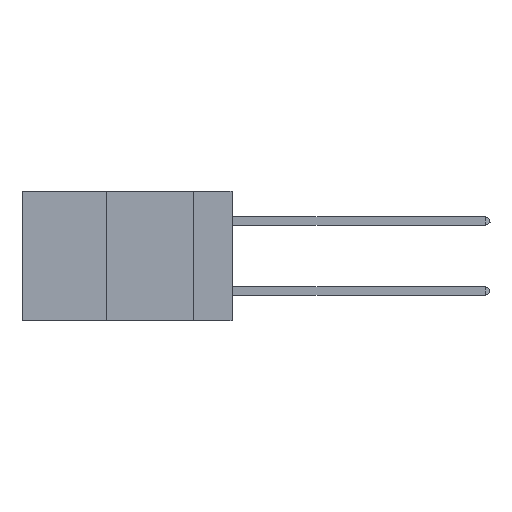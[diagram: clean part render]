
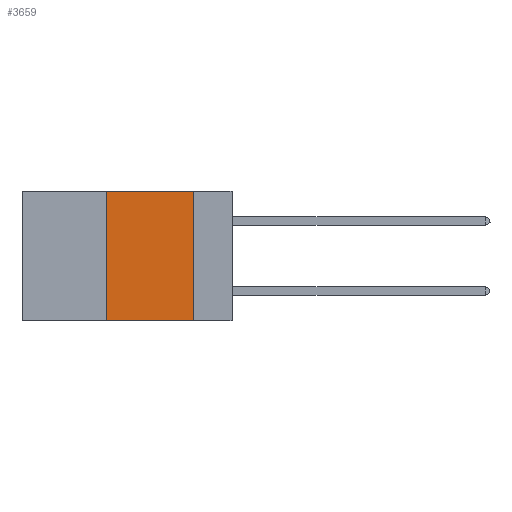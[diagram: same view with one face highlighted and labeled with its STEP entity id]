
A CAD part, left-side view. The second image highlights one B-rep face of the part: STEP entity #3659.
In plain terms, the highlighted planar face has unit normal (-1, 0, 0).
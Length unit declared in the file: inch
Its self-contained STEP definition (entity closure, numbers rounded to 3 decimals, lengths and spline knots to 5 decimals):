
#55 = CARTESIAN_POINT ( 'NONE',  ( 0., 0.36, 0. ) ) ;
#167 = CARTESIAN_POINT ( 'NONE',  ( 0., 0.36, -0.37 ) ) ;
#631 = VECTOR ( 'NONE', #4534, 39.37008 ) ;
#1031 = LINE ( 'NONE', #7110, #6328 ) ;
#2085 = VERTEX_POINT ( 'NONE', #4682 ) ;
#2636 = DIRECTION ( 'NONE',  ( 1., 0., 0. ) ) ;
#3373 = EDGE_CURVE ( 'NONE', #2085, #13718, #8470, .T. ) ;
#3577 = DIRECTION ( 'NONE',  ( 0., -1., 0. ) ) ;
#3659 = ADVANCED_FACE ( 'NONE', ( #12554 ), #13416, .F. ) ;
#4495 = ORIENTED_EDGE ( 'NONE', *, *, #4557, .F. ) ;
#4534 = DIRECTION ( 'NONE',  ( 0., 0., 1. ) ) ;
#4557 = EDGE_CURVE ( 'NONE', #13718, #7057, #9255, .T. ) ;
#4682 = CARTESIAN_POINT ( 'NONE',  ( 0., 0.36, 0. ) ) ;
#4752 = DIRECTION ( 'NONE',  ( 0., 0., -1. ) ) ;
#4755 = ORIENTED_EDGE ( 'NONE', *, *, #11218, .T. ) ;
#5039 = ORIENTED_EDGE ( 'NONE', *, *, #3373, .F. ) ;
#5550 = VERTEX_POINT ( 'NONE', #167 ) ;
#5906 = CARTESIAN_POINT ( 'NONE',  ( 0., 0.6, 0. ) ) ;
#6328 = VECTOR ( 'NONE', #3577, 39.37008 ) ;
#6916 = DIRECTION ( 'NONE',  ( 0., 0., -1. ) ) ;
#6926 = ORIENTED_EDGE ( 'NONE', *, *, #13237, .F. ) ;
#7057 = VERTEX_POINT ( 'NONE', #9154 ) ;
#7110 = CARTESIAN_POINT ( 'NONE',  ( 0., 0.6, -0.37 ) ) ;
#7448 = VECTOR ( 'NONE', #4752, 39.37008 ) ;
#8121 = VECTOR ( 'NONE', #8315, 39.37008 ) ;
#8315 = DIRECTION ( 'NONE',  ( 0., -1., 0. ) ) ;
#8470 = LINE ( 'NONE', #12751, #8121 ) ;
#9154 = CARTESIAN_POINT ( 'NONE',  ( 0., 0.11, -0.37 ) ) ;
#9255 = LINE ( 'NONE', #10183, #7448 ) ;
#9571 = EDGE_LOOP ( 'NONE', ( #4495, #5039, #6926, #4755 ) ) ;
#10183 = CARTESIAN_POINT ( 'NONE',  ( 0., 0.11, 0. ) ) ;
#11218 = EDGE_CURVE ( 'NONE', #5550, #7057, #1031, .T. ) ;
#11955 = AXIS2_PLACEMENT_3D ( 'NONE', #5906, #2636, #6916 ) ;
#12024 = CARTESIAN_POINT ( 'NONE',  ( 0., 0.11, 0. ) ) ;
#12554 = FACE_OUTER_BOUND ( 'NONE', #9571, .T. ) ;
#12751 = CARTESIAN_POINT ( 'NONE',  ( 0., 0.6, 0. ) ) ;
#13237 = EDGE_CURVE ( 'NONE', #5550, #2085, #14111, .T. ) ;
#13416 = PLANE ( 'NONE',  #11955 ) ;
#13718 = VERTEX_POINT ( 'NONE', #12024 ) ;
#14111 = LINE ( 'NONE', #55, #631 ) ;
